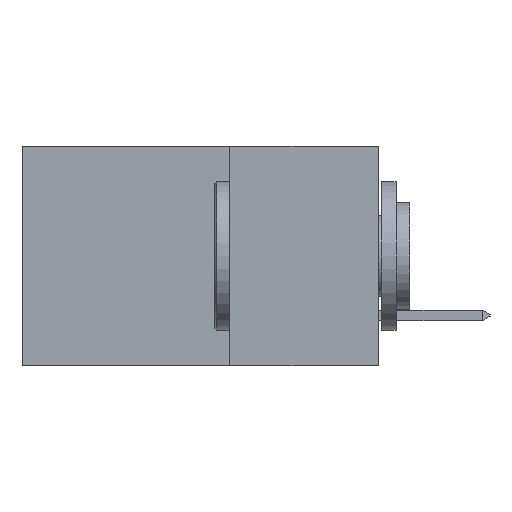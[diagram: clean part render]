
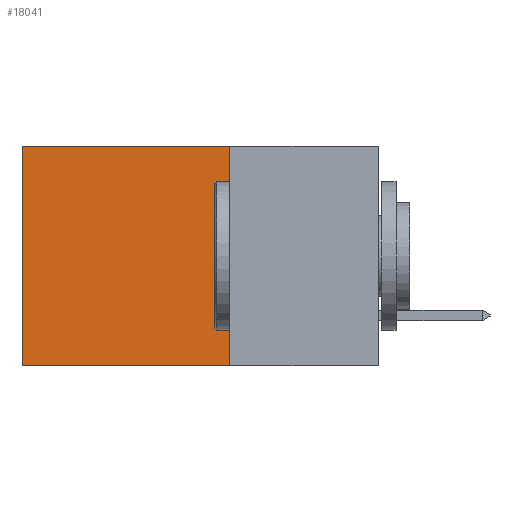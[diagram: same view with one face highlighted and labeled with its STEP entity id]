
A CAD part, left-side view. The second image highlights one B-rep face of the part: STEP entity #18041.
In plain terms, the highlighted planar face has unit normal (-1, 0, 0).
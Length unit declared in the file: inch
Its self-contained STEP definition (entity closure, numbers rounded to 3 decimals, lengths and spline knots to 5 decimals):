
#351 = DIRECTION ( 'NONE',  ( 0., 1., 0. ) ) ;
#610 = LINE ( 'NONE', #15595, #27551 ) ;
#1007 = CARTESIAN_POINT ( 'NONE',  ( 0.298, 0.25, 0. ) ) ;
#2790 = EDGE_LOOP ( 'NONE', ( #17282, #12154, #4590, #28490 ) ) ;
#4590 = ORIENTED_EDGE ( 'NONE', *, *, #28660, .F. ) ;
#4866 = DIRECTION ( 'NONE',  ( 0., 0., -1. ) ) ;
#5588 = FACE_OUTER_BOUND ( 'NONE', #2790, .T. ) ;
#6881 = VECTOR ( 'NONE', #31499, 39.37008 ) ;
#7876 = CARTESIAN_POINT ( 'NONE',  ( 0.298, 0.6, 0. ) ) ;
#8265 = VERTEX_POINT ( 'NONE', #7876 ) ;
#8682 = CARTESIAN_POINT ( 'NONE',  ( 0.298, 0.25, -0.37 ) ) ;
#9982 = CARTESIAN_POINT ( 'NONE',  ( 0.298, 0.6, 0. ) ) ;
#10164 = EDGE_CURVE ( 'NONE', #8265, #21250, #15164, .T. ) ;
#12130 = DIRECTION ( 'NONE',  ( 1., 0., 0. ) ) ;
#12154 = ORIENTED_EDGE ( 'NONE', *, *, #20799, .F. ) ;
#12250 = CARTESIAN_POINT ( 'NONE',  ( 0.298, 0.6, -0.37 ) ) ;
#14671 = VECTOR ( 'NONE', #26392, 39.37008 ) ;
#15164 = LINE ( 'NONE', #9982, #27721 ) ;
#15257 = LINE ( 'NONE', #26593, #6881 ) ;
#15595 = CARTESIAN_POINT ( 'NONE',  ( 0.298, 0.25, -0.37 ) ) ;
#17282 = ORIENTED_EDGE ( 'NONE', *, *, #10164, .T. ) ;
#18041 = ADVANCED_FACE ( 'NONE', ( #5588 ), #32022, .F. ) ;
#20514 = AXIS2_PLACEMENT_3D ( 'NONE', #27213, #12130, #29653 ) ;
#20799 = EDGE_CURVE ( 'NONE', #21005, #21250, #610, .T. ) ;
#21005 = VERTEX_POINT ( 'NONE', #8682 ) ;
#21250 = VERTEX_POINT ( 'NONE', #12250 ) ;
#22697 = CARTESIAN_POINT ( 'NONE',  ( 0.298, 0.25, 0. ) ) ;
#22946 = EDGE_CURVE ( 'NONE', #27706, #8265, #15257, .T. ) ;
#26392 = DIRECTION ( 'NONE',  ( 0., 0., -1. ) ) ;
#26593 = CARTESIAN_POINT ( 'NONE',  ( 0.298, 0.25, 0. ) ) ;
#27213 = CARTESIAN_POINT ( 'NONE',  ( 0.298, 0.25, 0. ) ) ;
#27551 = VECTOR ( 'NONE', #351, 39.37008 ) ;
#27706 = VERTEX_POINT ( 'NONE', #22697 ) ;
#27721 = VECTOR ( 'NONE', #4866, 39.37008 ) ;
#28023 = LINE ( 'NONE', #1007, #14671 ) ;
#28490 = ORIENTED_EDGE ( 'NONE', *, *, #22946, .T. ) ;
#28660 = EDGE_CURVE ( 'NONE', #27706, #21005, #28023, .T. ) ;
#29653 = DIRECTION ( 'NONE',  ( 0., 0., -1. ) ) ;
#31499 = DIRECTION ( 'NONE',  ( 0., 1., 0. ) ) ;
#32022 = PLANE ( 'NONE',  #20514 ) ;
